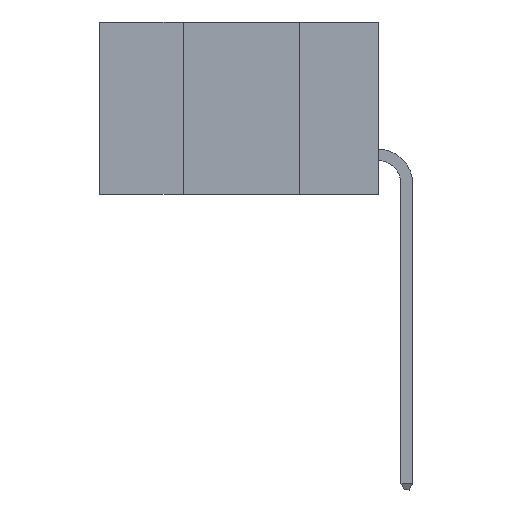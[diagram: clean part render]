
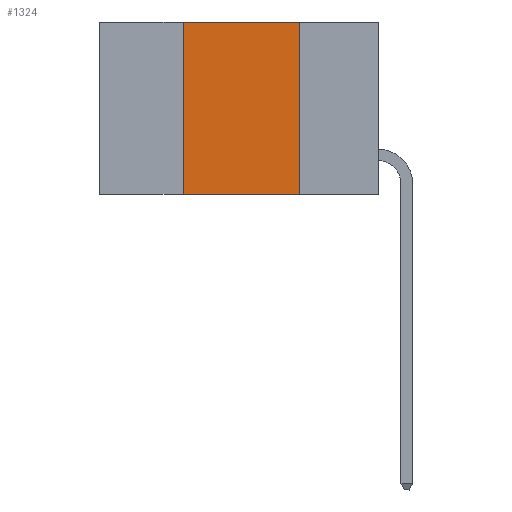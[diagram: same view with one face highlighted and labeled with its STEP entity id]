
A CAD part, left-side view. The second image highlights one B-rep face of the part: STEP entity #1324.
In plain terms, the highlighted planar face has unit normal (-1, 0, 0).
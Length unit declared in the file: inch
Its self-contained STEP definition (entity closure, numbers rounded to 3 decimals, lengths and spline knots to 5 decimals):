
#220 = LINE ( 'NONE', #2985, #2107 ) ;
#371 = CARTESIAN_POINT ( 'NONE',  ( 0., 0.42, 0. ) ) ;
#381 = VERTEX_POINT ( 'NONE', #1470 ) ;
#535 = CARTESIAN_POINT ( 'NONE',  ( 0., 0.6, 0. ) ) ;
#565 = DIRECTION ( 'NONE',  ( 0., 0., -1. ) ) ;
#726 = ORIENTED_EDGE ( 'NONE', *, *, #6251, .F. ) ;
#1324 = ADVANCED_FACE ( 'NONE', ( #3002 ), #5153, .F. ) ;
#1380 = DIRECTION ( 'NONE',  ( 1., 0., 0. ) ) ;
#1435 = ORIENTED_EDGE ( 'NONE', *, *, #5263, .F. ) ;
#1470 = CARTESIAN_POINT ( 'NONE',  ( 0., 0.17, -0.37 ) ) ;
#1620 = VERTEX_POINT ( 'NONE', #6084 ) ;
#1882 = LINE ( 'NONE', #7740, #9176 ) ;
#2107 = VECTOR ( 'NONE', #6268, 39.37008 ) ;
#2726 = VERTEX_POINT ( 'NONE', #371 ) ;
#2802 = DIRECTION ( 'NONE',  ( 0., -1., 0. ) ) ;
#2985 = CARTESIAN_POINT ( 'NONE',  ( 0., 0.42, 0. ) ) ;
#3002 = FACE_OUTER_BOUND ( 'NONE', #8198, .T. ) ;
#3069 = VECTOR ( 'NONE', #2802, 39.37008 ) ;
#3294 = LINE ( 'NONE', #9083, #3069 ) ;
#4360 = ORIENTED_EDGE ( 'NONE', *, *, #4399, .T. ) ;
#4399 = EDGE_CURVE ( 'NONE', #5660, #381, #1882, .T. ) ;
#5153 = PLANE ( 'NONE',  #9336 ) ;
#5252 = ORIENTED_EDGE ( 'NONE', *, *, #8511, .F. ) ;
#5263 = EDGE_CURVE ( 'NONE', #5660, #2726, #220, .T. ) ;
#5660 = VERTEX_POINT ( 'NONE', #7166 ) ;
#5930 = VECTOR ( 'NONE', #565, 39.37008 ) ;
#6084 = CARTESIAN_POINT ( 'NONE',  ( 0., 0.17, 0. ) ) ;
#6251 = EDGE_CURVE ( 'NONE', #1620, #381, #7113, .T. ) ;
#6268 = DIRECTION ( 'NONE',  ( 0., 0., 1. ) ) ;
#6561 = DIRECTION ( 'NONE',  ( 0., 0., -1. ) ) ;
#7113 = LINE ( 'NONE', #9185, #5930 ) ;
#7166 = CARTESIAN_POINT ( 'NONE',  ( 0., 0.42, -0.37 ) ) ;
#7735 = DIRECTION ( 'NONE',  ( 0., -1., 0. ) ) ;
#7740 = CARTESIAN_POINT ( 'NONE',  ( 0., 0.6, -0.37 ) ) ;
#8198 = EDGE_LOOP ( 'NONE', ( #726, #5252, #1435, #4360 ) ) ;
#8511 = EDGE_CURVE ( 'NONE', #2726, #1620, #3294, .T. ) ;
#9083 = CARTESIAN_POINT ( 'NONE',  ( 0., 0.6, 0. ) ) ;
#9176 = VECTOR ( 'NONE', #7735, 39.37008 ) ;
#9185 = CARTESIAN_POINT ( 'NONE',  ( 0., 0.17, 0. ) ) ;
#9336 = AXIS2_PLACEMENT_3D ( 'NONE', #535, #1380, #6561 ) ;
